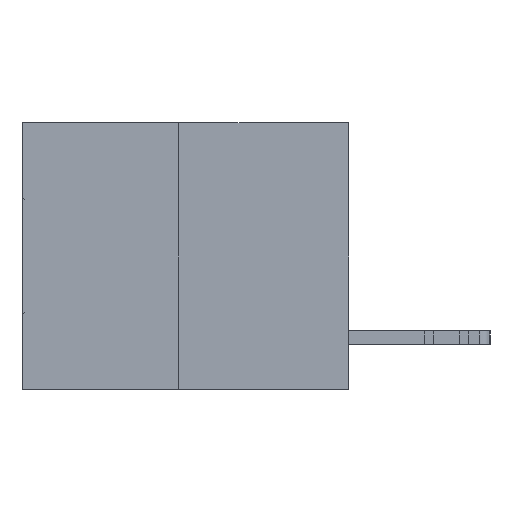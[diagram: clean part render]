
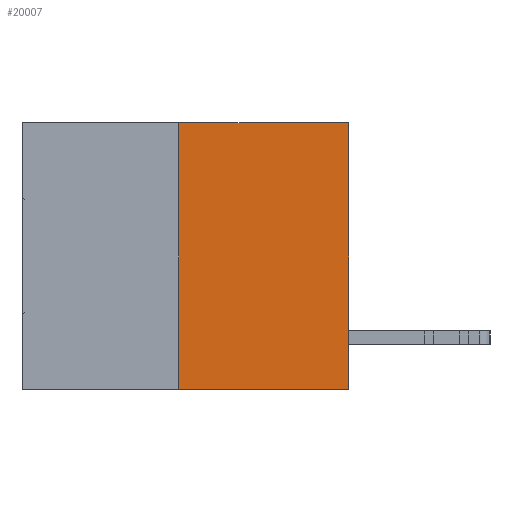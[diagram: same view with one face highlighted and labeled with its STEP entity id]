
A CAD part, left-side view. The second image highlights one B-rep face of the part: STEP entity #20007.
In plain terms, the highlighted planar face has unit normal (-1, 0, 0).
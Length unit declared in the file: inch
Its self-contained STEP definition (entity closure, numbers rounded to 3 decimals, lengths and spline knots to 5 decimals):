
#1092 = EDGE_LOOP ( 'NONE', ( #28980, #18004, #17297, #11790 ) ) ;
#1569 = DIRECTION ( 'NONE',  ( 0., -1., 0. ) ) ;
#2397 = LINE ( 'NONE', #6985, #29914 ) ;
#3577 = FACE_OUTER_BOUND ( 'NONE', #1092, .T. ) ;
#6985 = CARTESIAN_POINT ( 'NONE',  ( 0., 0.6, 0. ) ) ;
#8078 = VECTOR ( 'NONE', #31995, 39.37008 ) ;
#11034 = CARTESIAN_POINT ( 'NONE',  ( 0., 0.312, -0.49 ) ) ;
#11308 = EDGE_CURVE ( 'NONE', #25697, #32424, #2397, .T. ) ;
#11604 = EDGE_CURVE ( 'NONE', #22699, #19644, #29003, .T. ) ;
#11790 = ORIENTED_EDGE ( 'NONE', *, *, #11308, .F. ) ;
#12523 = CARTESIAN_POINT ( 'NONE',  ( 0., 0., 0. ) ) ;
#12863 = CARTESIAN_POINT ( 'NONE',  ( 0., 0.312, -0.49 ) ) ;
#13042 = EDGE_CURVE ( 'NONE', #19644, #32424, #18225, .T. ) ;
#13748 = DIRECTION ( 'NONE',  ( 0., 0., 1. ) ) ;
#14944 = DIRECTION ( 'NONE',  ( 1., 0., 0. ) ) ;
#17297 = ORIENTED_EDGE ( 'NONE', *, *, #13042, .T. ) ;
#18004 = ORIENTED_EDGE ( 'NONE', *, *, #11604, .T. ) ;
#18225 = LINE ( 'NONE', #31086, #26427 ) ;
#19644 = VERTEX_POINT ( 'NONE', #31220 ) ;
#19756 = VECTOR ( 'NONE', #13748, 39.37008 ) ;
#20007 = ADVANCED_FACE ( 'NONE', ( #3577 ), #30830, .F. ) ;
#20551 = LINE ( 'NONE', #11034, #19756 ) ;
#21365 = AXIS2_PLACEMENT_3D ( 'NONE', #22427, #14944, #25546 ) ;
#22427 = CARTESIAN_POINT ( 'NONE',  ( 0., 0.6, 0. ) ) ;
#22699 = VERTEX_POINT ( 'NONE', #12863 ) ;
#23771 = CARTESIAN_POINT ( 'NONE',  ( 0., 0.312, 0. ) ) ;
#25546 = DIRECTION ( 'NONE',  ( 0., 0., -1. ) ) ;
#25697 = VERTEX_POINT ( 'NONE', #23771 ) ;
#26206 = CARTESIAN_POINT ( 'NONE',  ( 0., 0.6, -0.49 ) ) ;
#26427 = VECTOR ( 'NONE', #33598, 39.37008 ) ;
#28980 = ORIENTED_EDGE ( 'NONE', *, *, #33335, .F. ) ;
#29003 = LINE ( 'NONE', #26206, #8078 ) ;
#29914 = VECTOR ( 'NONE', #1569, 39.37008 ) ;
#30830 = PLANE ( 'NONE',  #21365 ) ;
#31086 = CARTESIAN_POINT ( 'NONE',  ( 0., 0., 0. ) ) ;
#31220 = CARTESIAN_POINT ( 'NONE',  ( 0., 0., -0.49 ) ) ;
#31995 = DIRECTION ( 'NONE',  ( 0., -1., 0. ) ) ;
#32424 = VERTEX_POINT ( 'NONE', #12523 ) ;
#33335 = EDGE_CURVE ( 'NONE', #22699, #25697, #20551, .T. ) ;
#33598 = DIRECTION ( 'NONE',  ( 0., 0., 1. ) ) ;
